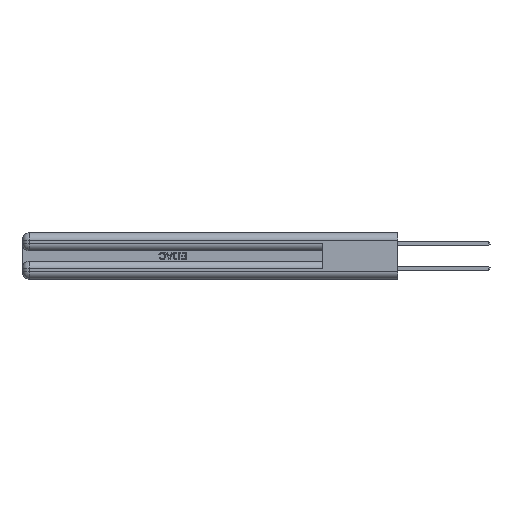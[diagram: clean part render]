
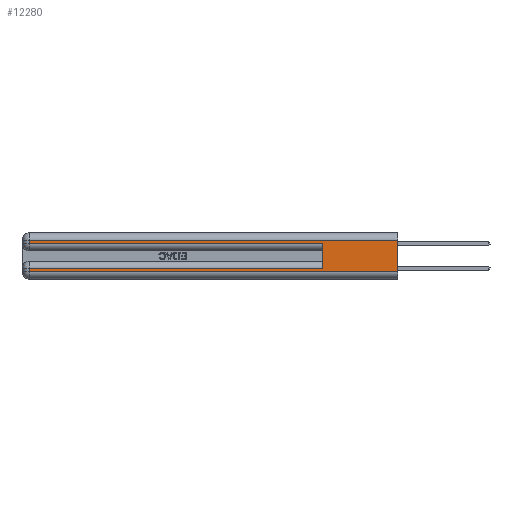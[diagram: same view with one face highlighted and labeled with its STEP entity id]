
A CAD part, left-side view. The second image highlights one B-rep face of the part: STEP entity #12280.
In plain terms, the highlighted planar face has unit normal (-1, 0, 0).
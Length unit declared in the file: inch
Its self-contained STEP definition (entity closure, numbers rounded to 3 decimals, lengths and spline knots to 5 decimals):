
#1526 = LINE ( 'NONE', #19992, #14611 ) ;
#1537 = VECTOR ( 'NONE', #20589, 39.37008 ) ;
#2796 = LINE ( 'NONE', #4739, #1537 ) ;
#3685 = EDGE_CURVE ( 'NONE', #49785, #11575, #42208, .T. ) ;
#3923 = EDGE_CURVE ( 'NONE', #19469, #49785, #50905, .T. ) ;
#4566 = ORIENTED_EDGE ( 'NONE', *, *, #15666, .T. ) ;
#4739 = CARTESIAN_POINT ( 'NONE',  ( 0., 0., 0.31 ) ) ;
#4744 = EDGE_CURVE ( 'NONE', #37815, #13784, #1526, .T. ) ;
#5766 = CARTESIAN_POINT ( 'NONE',  ( 0., 2.94, 0.31 ) ) ;
#5926 = ORIENTED_EDGE ( 'NONE', *, *, #3685, .T. ) ;
#8103 = ORIENTED_EDGE ( 'NONE', *, *, #10907, .T. ) ;
#9617 = DIRECTION ( 'NONE',  ( 0., 1., 0. ) ) ;
#10907 = EDGE_CURVE ( 'NONE', #41059, #51033, #13800, .T. ) ;
#11575 = VERTEX_POINT ( 'NONE', #18987 ) ;
#12280 = ADVANCED_FACE ( 'NONE', ( #34395 ), #35803, .F. ) ;
#13784 = VERTEX_POINT ( 'NONE', #48550 ) ;
#13800 = LINE ( 'NONE', #17678, #33819 ) ;
#14486 = DIRECTION ( 'NONE',  ( 0., 0., -1. ) ) ;
#14611 = VECTOR ( 'NONE', #47926, 39.37008 ) ;
#15666 = EDGE_CURVE ( 'NONE', #51033, #37815, #17131, .T. ) ;
#15874 = DIRECTION ( 'NONE',  ( 1., 0., 0. ) ) ;
#16155 = VECTOR ( 'NONE', #17723, 39.37008 ) ;
#17131 = LINE ( 'NONE', #47305, #37163 ) ;
#17577 = ORIENTED_EDGE ( 'NONE', *, *, #32241, .F. ) ;
#17678 = CARTESIAN_POINT ( 'NONE',  ( 0., 0., 0.085 ) ) ;
#17723 = DIRECTION ( 'NONE',  ( 0., 0., -1. ) ) ;
#18987 = CARTESIAN_POINT ( 'NONE',  ( 0., 0.6, 0.285 ) ) ;
#19469 = VERTEX_POINT ( 'NONE', #5766 ) ;
#19992 = CARTESIAN_POINT ( 'NONE',  ( 0., 0., 0.06 ) ) ;
#20589 = DIRECTION ( 'NONE',  ( 0., 1., 0. ) ) ;
#22337 = CARTESIAN_POINT ( 'NONE',  ( 0., 2.94, 0.37 ) ) ;
#22606 = CARTESIAN_POINT ( 'NONE',  ( 0., 2.94, 0.085 ) ) ;
#24613 = DIRECTION ( 'NONE',  ( 0., 0., 1. ) ) ;
#25988 = VECTOR ( 'NONE', #24613, 39.37008 ) ;
#26845 = CARTESIAN_POINT ( 'NONE',  ( 0., 0.6, 0.085 ) ) ;
#28198 = EDGE_CURVE ( 'NONE', #49860, #19469, #2796, .T. ) ;
#29010 = DIRECTION ( 'NONE',  ( 0., -1., 0. ) ) ;
#29547 = AXIS2_PLACEMENT_3D ( 'NONE', #39806, #15874, #43770 ) ;
#29941 = ORIENTED_EDGE ( 'NONE', *, *, #36266, .F. ) ;
#29955 = CARTESIAN_POINT ( 'NONE',  ( 0., 2.94, 0.06 ) ) ;
#31625 = VECTOR ( 'NONE', #29010, 39.37008 ) ;
#32003 = CARTESIAN_POINT ( 'NONE',  ( 0., 2.94, 0.285 ) ) ;
#32241 = EDGE_CURVE ( 'NONE', #49860, #13784, #46759, .T. ) ;
#33819 = VECTOR ( 'NONE', #9617, 39.37008 ) ;
#34395 = FACE_OUTER_BOUND ( 'NONE', #47913, .T. ) ;
#35803 = PLANE ( 'NONE',  #29547 ) ;
#36266 = EDGE_CURVE ( 'NONE', #41059, #11575, #36657, .T. ) ;
#36657 = LINE ( 'NONE', #40376, #25988 ) ;
#37163 = VECTOR ( 'NONE', #51270, 39.37008 ) ;
#37815 = VERTEX_POINT ( 'NONE', #29955 ) ;
#38470 = ORIENTED_EDGE ( 'NONE', *, *, #4744, .T. ) ;
#39806 = CARTESIAN_POINT ( 'NONE',  ( 0., 0., 0.37 ) ) ;
#40331 = VECTOR ( 'NONE', #14486, 39.37008 ) ;
#40376 = CARTESIAN_POINT ( 'NONE',  ( 0., 0.6, 0.145 ) ) ;
#41059 = VERTEX_POINT ( 'NONE', #26845 ) ;
#41621 = CARTESIAN_POINT ( 'NONE',  ( 0., 0., 0.37 ) ) ;
#42208 = LINE ( 'NONE', #45054, #31625 ) ;
#43770 = DIRECTION ( 'NONE',  ( 0., 0., -1. ) ) ;
#45054 = CARTESIAN_POINT ( 'NONE',  ( 0., 0., 0.285 ) ) ;
#46759 = LINE ( 'NONE', #41621, #16155 ) ;
#47305 = CARTESIAN_POINT ( 'NONE',  ( 0., 2.94, 0.37 ) ) ;
#47836 = ORIENTED_EDGE ( 'NONE', *, *, #28198, .T. ) ;
#47913 = EDGE_LOOP ( 'NONE', ( #17577, #47836, #48669, #5926, #29941, #8103, #4566, #38470 ) ) ;
#47926 = DIRECTION ( 'NONE',  ( 0., -1., 0. ) ) ;
#48373 = CARTESIAN_POINT ( 'NONE',  ( 0., 0., 0.31 ) ) ;
#48550 = CARTESIAN_POINT ( 'NONE',  ( 0., 0., 0.06 ) ) ;
#48669 = ORIENTED_EDGE ( 'NONE', *, *, #3923, .T. ) ;
#49785 = VERTEX_POINT ( 'NONE', #32003 ) ;
#49860 = VERTEX_POINT ( 'NONE', #48373 ) ;
#50905 = LINE ( 'NONE', #22337, #40331 ) ;
#51033 = VERTEX_POINT ( 'NONE', #22606 ) ;
#51270 = DIRECTION ( 'NONE',  ( 0., 0., -1. ) ) ;
